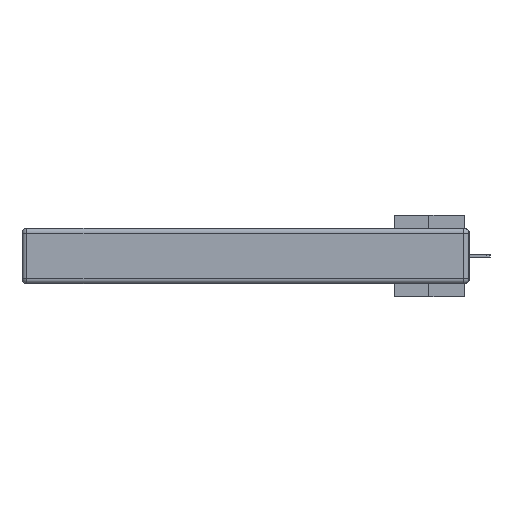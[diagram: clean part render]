
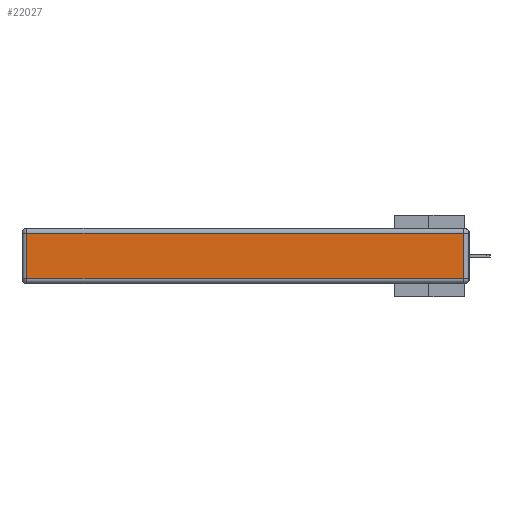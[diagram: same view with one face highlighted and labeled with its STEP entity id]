
A CAD part, left-side view. The second image highlights one B-rep face of the part: STEP entity #22027.
In plain terms, the highlighted planar face has unit normal (-1, 0, 0).
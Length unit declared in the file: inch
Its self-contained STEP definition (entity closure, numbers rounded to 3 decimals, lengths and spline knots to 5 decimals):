
#566 = LINE ( 'NONE', #13608, #10139 ) ;
#1029 = EDGE_CURVE ( 'NONE', #34017, #2580, #16490, .T. ) ;
#2580 = VERTEX_POINT ( 'NONE', #16861 ) ;
#2762 = LINE ( 'NONE', #15188, #37932 ) ;
#5298 = CARTESIAN_POINT ( 'NONE',  ( 0., 0.03, -0.03 ) ) ;
#6756 = DIRECTION ( 'NONE',  ( 0., 1., 0. ) ) ;
#9846 = VERTEX_POINT ( 'NONE', #31646 ) ;
#10139 = VECTOR ( 'NONE', #16751, 39.37008 ) ;
#12825 = DIRECTION ( 'NONE',  ( 0., 0., 1. ) ) ;
#13600 = DIRECTION ( 'NONE',  ( 0., 0., 1. ) ) ;
#13608 = CARTESIAN_POINT ( 'NONE',  ( 0., 2.72, -0.343 ) ) ;
#14832 = ORIENTED_EDGE ( 'NONE', *, *, #29985, .T. ) ;
#15188 = CARTESIAN_POINT ( 'NONE',  ( 0., 0., -0.313 ) ) ;
#15598 = AXIS2_PLACEMENT_3D ( 'NONE', #26717, #19867, #13600 ) ;
#16490 = LINE ( 'NONE', #38746, #20071 ) ;
#16751 = DIRECTION ( 'NONE',  ( 0., 0., -1. ) ) ;
#16861 = CARTESIAN_POINT ( 'NONE',  ( 0., 2.72, -0.03 ) ) ;
#16953 = CARTESIAN_POINT ( 'NONE',  ( 0., 0.03, -0.313 ) ) ;
#19563 = VECTOR ( 'NONE', #12825, 39.37008 ) ;
#19867 = DIRECTION ( 'NONE',  ( -1., 0., 0. ) ) ;
#20071 = VECTOR ( 'NONE', #6756, 39.37008 ) ;
#20165 = EDGE_CURVE ( 'NONE', #20751, #34017, #22001, .T. ) ;
#20751 = VERTEX_POINT ( 'NONE', #16953 ) ;
#22001 = LINE ( 'NONE', #40923, #19563 ) ;
#22027 = ADVANCED_FACE ( 'NONE', ( #29417 ), #29838, .T. ) ;
#22515 = ORIENTED_EDGE ( 'NONE', *, *, #1029, .T. ) ;
#23607 = ORIENTED_EDGE ( 'NONE', *, *, #33729, .T. ) ;
#26717 = CARTESIAN_POINT ( 'NONE',  ( 0., 0., -0.343 ) ) ;
#29417 = FACE_OUTER_BOUND ( 'NONE', #29905, .T. ) ;
#29838 = PLANE ( 'NONE',  #15598 ) ;
#29905 = EDGE_LOOP ( 'NONE', ( #14832, #35428, #22515, #23607 ) ) ;
#29985 = EDGE_CURVE ( 'NONE', #9846, #20751, #2762, .T. ) ;
#31646 = CARTESIAN_POINT ( 'NONE',  ( 0., 2.72, -0.313 ) ) ;
#33729 = EDGE_CURVE ( 'NONE', #2580, #9846, #566, .T. ) ;
#34017 = VERTEX_POINT ( 'NONE', #5298 ) ;
#35428 = ORIENTED_EDGE ( 'NONE', *, *, #20165, .T. ) ;
#37860 = DIRECTION ( 'NONE',  ( 0., -1., 0. ) ) ;
#37932 = VECTOR ( 'NONE', #37860, 39.37008 ) ;
#38746 = CARTESIAN_POINT ( 'NONE',  ( 0., 2.75, -0.03 ) ) ;
#40923 = CARTESIAN_POINT ( 'NONE',  ( 0., 0.03, -0.343 ) ) ;
